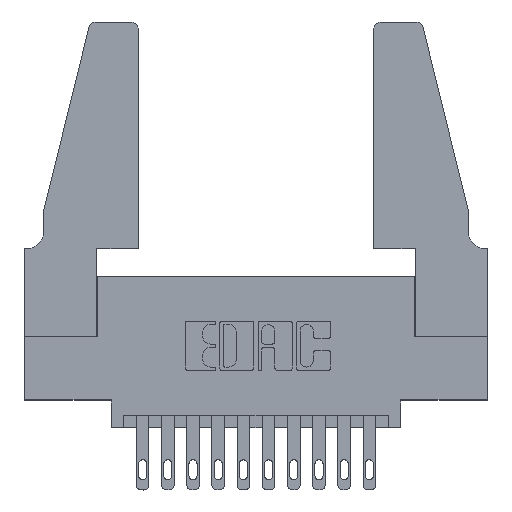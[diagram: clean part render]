
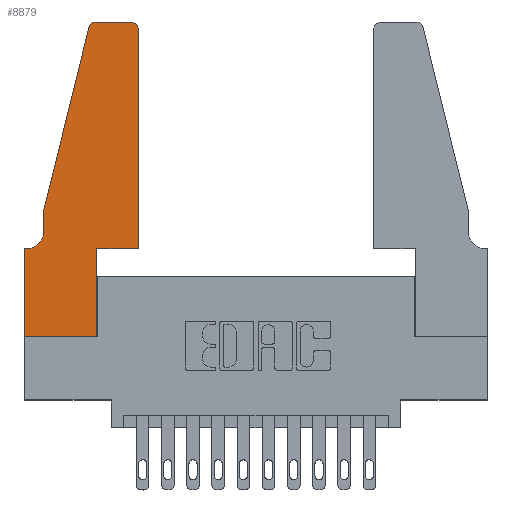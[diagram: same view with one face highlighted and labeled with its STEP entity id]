
A CAD part, top view. The second image highlights one B-rep face of the part: STEP entity #8879.
In plain terms, the highlighted planar face has unit normal (0, 0, 1).
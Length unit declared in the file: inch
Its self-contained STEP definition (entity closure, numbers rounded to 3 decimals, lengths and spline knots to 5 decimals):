
#129 = DIRECTION ( 'NONE',  ( 1., 0., 0. ) ) ;
#432 = ORIENTED_EDGE ( 'NONE', *, *, #4252, .T. ) ;
#487 = AXIS2_PLACEMENT_3D ( 'NONE', #4033, #12795, #2748 ) ;
#547 = DIRECTION ( 'NONE',  ( 0., 1., 0. ) ) ;
#603 = EDGE_CURVE ( 'NONE', #10500, #12027, #8892, .T. ) ;
#815 = EDGE_CURVE ( 'NONE', #13994, #10500, #8186, .T. ) ;
#1023 = DIRECTION ( 'NONE',  ( 1., 0., 0. ) ) ;
#1066 = ORIENTED_EDGE ( 'NONE', *, *, #603, .T. ) ;
#1330 = EDGE_LOOP ( 'NONE', ( #12595, #14325, #12293, #7953, #8117, #1955, #1066, #6799, #4983, #5718, #432, #7857 ) ) ;
#1415 = CARTESIAN_POINT ( 'NONE',  ( 0., 0.35, 0.37 ) ) ;
#1461 = DIRECTION ( 'NONE',  ( 1., 0., 0. ) ) ;
#1580 = AXIS2_PLACEMENT_3D ( 'NONE', #13001, #5401, #8367 ) ;
#1755 = VECTOR ( 'NONE', #129, 39.37008 ) ;
#1867 = AXIS2_PLACEMENT_3D ( 'NONE', #1415, #2544, #1461 ) ;
#1949 = VERTEX_POINT ( 'NONE', #13239 ) ;
#1955 = ORIENTED_EDGE ( 'NONE', *, *, #815, .T. ) ;
#1992 = CARTESIAN_POINT ( 'NONE',  ( 0.0055, 0.35, 0.37 ) ) ;
#2019 = DIRECTION ( 'NONE',  ( 0., 0., 1. ) ) ;
#2523 = CIRCLE ( 'NONE', #1580, 0.07 ) ;
#2544 = DIRECTION ( 'NONE',  ( 0., 0., 1. ) ) ;
#2572 = DIRECTION ( 'NONE',  ( -0.239, -0.971, 0. ) ) ;
#2748 = DIRECTION ( 'NONE',  ( 1., 0., 0. ) ) ;
#2934 = AXIS2_PLACEMENT_3D ( 'NONE', #13220, #2019, #1023 ) ;
#3218 = VECTOR ( 'NONE', #11597, 39.37008 ) ;
#3270 = CARTESIAN_POINT ( 'NONE',  ( 0.4505, 1.22, 0.37 ) ) ;
#3633 = VECTOR ( 'NONE', #4904, 39.37008 ) ;
#3691 = EDGE_CURVE ( 'NONE', #12027, #8774, #12449, .T. ) ;
#3708 = CARTESIAN_POINT ( 'NONE',  ( 0.0755, 0.42, 0.37 ) ) ;
#3979 = CARTESIAN_POINT ( 'NONE',  ( 0.0755, 0.5, 0.37 ) ) ;
#4033 = CARTESIAN_POINT ( 'NONE',  ( 0.284, 1.22, 0.37 ) ) ;
#4252 = EDGE_CURVE ( 'NONE', #13866, #10276, #12106, .T. ) ;
#4449 = VERTEX_POINT ( 'NONE', #13378 ) ;
#4904 = DIRECTION ( 'NONE',  ( 0., -1., 0. ) ) ;
#4983 = ORIENTED_EDGE ( 'NONE', *, *, #10528, .T. ) ;
#5201 = VERTEX_POINT ( 'NONE', #5656 ) ;
#5401 = DIRECTION ( 'NONE',  ( 0., 0., -1. ) ) ;
#5414 = CARTESIAN_POINT ( 'NONE',  ( 0., 0., 0.37 ) ) ;
#5534 = VECTOR ( 'NONE', #11589, 39.37008 ) ;
#5654 = DIRECTION ( 'NONE',  ( 0., -1., 0. ) ) ;
#5656 = CARTESIAN_POINT ( 'NONE',  ( 0.0755, 0.5, 0.37 ) ) ;
#5702 = CARTESIAN_POINT ( 'NONE',  ( 0.0755, 0.35, 0.37 ) ) ;
#5718 = ORIENTED_EDGE ( 'NONE', *, *, #11643, .T. ) ;
#5868 = PLANE ( 'NONE',  #1867 ) ;
#5978 = CIRCLE ( 'NONE', #2934, 0.03 ) ;
#6017 = CARTESIAN_POINT ( 'NONE',  ( 0., 0.35, 0.37 ) ) ;
#6303 = VERTEX_POINT ( 'NONE', #9485 ) ;
#6585 = CIRCLE ( 'NONE', #487, 0.03 ) ;
#6799 = ORIENTED_EDGE ( 'NONE', *, *, #3691, .T. ) ;
#6893 = EDGE_CURVE ( 'NONE', #12089, #1949, #12183, .T. ) ;
#7073 = CARTESIAN_POINT ( 'NONE',  ( 0., 0., 0.37 ) ) ;
#7688 = LINE ( 'NONE', #10346, #1755 ) ;
#7812 = DIRECTION ( 'NONE',  ( -1., 0., 0. ) ) ;
#7857 = ORIENTED_EDGE ( 'NONE', *, *, #10803, .T. ) ;
#7953 = ORIENTED_EDGE ( 'NONE', *, *, #8014, .T. ) ;
#8014 = EDGE_CURVE ( 'NONE', #5201, #14240, #12314, .T. ) ;
#8117 = ORIENTED_EDGE ( 'NONE', *, *, #9772, .T. ) ;
#8186 = LINE ( 'NONE', #5702, #12895 ) ;
#8299 = CARTESIAN_POINT ( 'NONE',  ( 0.4505, 0.35, 0.37 ) ) ;
#8367 = DIRECTION ( 'NONE',  ( -1., 0., 0. ) ) ;
#8543 = EDGE_CURVE ( 'NONE', #4449, #5201, #13318, .T. ) ;
#8774 = VERTEX_POINT ( 'NONE', #12092 ) ;
#8879 = ADVANCED_FACE ( 'NONE', ( #12628 ), #5868, .T. ) ;
#8892 = LINE ( 'NONE', #10035, #9757 ) ;
#9485 = CARTESIAN_POINT ( 'NONE',  ( 0.2865, 0.35, 0.37 ) ) ;
#9757 = VECTOR ( 'NONE', #5654, 39.37008 ) ;
#9772 = EDGE_CURVE ( 'NONE', #14240, #13994, #2523, .T. ) ;
#9960 = LINE ( 'NONE', #11455, #3218 ) ;
#10035 = CARTESIAN_POINT ( 'NONE',  ( 0., 0., 0.37 ) ) ;
#10276 = VERTEX_POINT ( 'NONE', #3270 ) ;
#10346 = CARTESIAN_POINT ( 'NONE',  ( 0.4505, 0.35, 0.37 ) ) ;
#10500 = VERTEX_POINT ( 'NONE', #6017 ) ;
#10528 = EDGE_CURVE ( 'NONE', #8774, #6303, #9960, .T. ) ;
#10728 = VECTOR ( 'NONE', #2572, 39.37008 ) ;
#10735 = CARTESIAN_POINT ( 'NONE',  ( 0.0755, 0.5, 0.37 ) ) ;
#10803 = EDGE_CURVE ( 'NONE', #10276, #12089, #5978, .T. ) ;
#11397 = VECTOR ( 'NONE', #547, 39.37008 ) ;
#11455 = CARTESIAN_POINT ( 'NONE',  ( 0.2865, 0.35, 0.37 ) ) ;
#11470 = VECTOR ( 'NONE', #12220, 39.37008 ) ;
#11589 = DIRECTION ( 'NONE',  ( 1., 0., 0. ) ) ;
#11597 = DIRECTION ( 'NONE',  ( 0., 1., 0. ) ) ;
#11643 = EDGE_CURVE ( 'NONE', #6303, #13866, #7688, .T. ) ;
#12027 = VERTEX_POINT ( 'NONE', #5414 ) ;
#12089 = VERTEX_POINT ( 'NONE', #13289 ) ;
#12092 = CARTESIAN_POINT ( 'NONE',  ( 0.2865, 0., 0.37 ) ) ;
#12106 = LINE ( 'NONE', #12716, #11397 ) ;
#12183 = LINE ( 'NONE', #13389, #11470 ) ;
#12220 = DIRECTION ( 'NONE',  ( -1., 0., 0. ) ) ;
#12293 = ORIENTED_EDGE ( 'NONE', *, *, #8543, .T. ) ;
#12314 = LINE ( 'NONE', #10735, #3633 ) ;
#12449 = LINE ( 'NONE', #7073, #5534 ) ;
#12595 = ORIENTED_EDGE ( 'NONE', *, *, #6893, .T. ) ;
#12628 = FACE_OUTER_BOUND ( 'NONE', #1330, .T. ) ;
#12716 = CARTESIAN_POINT ( 'NONE',  ( 0.4505, 0.35, 0.37 ) ) ;
#12795 = DIRECTION ( 'NONE',  ( 0., 0., 1. ) ) ;
#12895 = VECTOR ( 'NONE', #7812, 39.37008 ) ;
#13001 = CARTESIAN_POINT ( 'NONE',  ( 0.0055, 0.42, 0.37 ) ) ;
#13122 = EDGE_CURVE ( 'NONE', #1949, #4449, #6585, .T. ) ;
#13220 = CARTESIAN_POINT ( 'NONE',  ( 0.4205, 1.22, 0.37 ) ) ;
#13239 = CARTESIAN_POINT ( 'NONE',  ( 0.284, 1.25, 0.37 ) ) ;
#13289 = CARTESIAN_POINT ( 'NONE',  ( 0.4205, 1.25, 0.37 ) ) ;
#13318 = LINE ( 'NONE', #3979, #10728 ) ;
#13378 = CARTESIAN_POINT ( 'NONE',  ( 0.25487, 1.22718, 0.37 ) ) ;
#13389 = CARTESIAN_POINT ( 'NONE',  ( 0.2605, 1.25, 0.37 ) ) ;
#13866 = VERTEX_POINT ( 'NONE', #8299 ) ;
#13994 = VERTEX_POINT ( 'NONE', #1992 ) ;
#14240 = VERTEX_POINT ( 'NONE', #3708 ) ;
#14325 = ORIENTED_EDGE ( 'NONE', *, *, #13122, .T. ) ;
